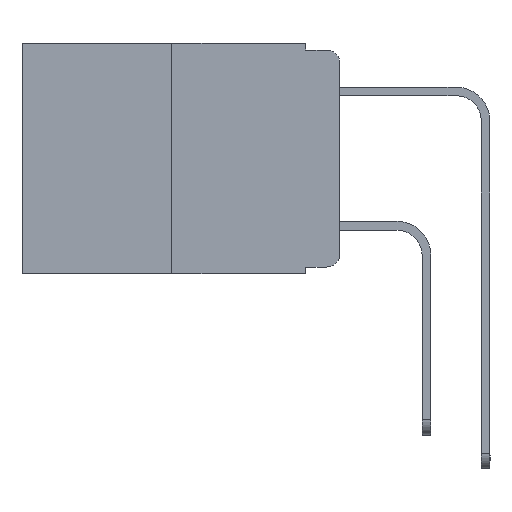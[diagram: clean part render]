
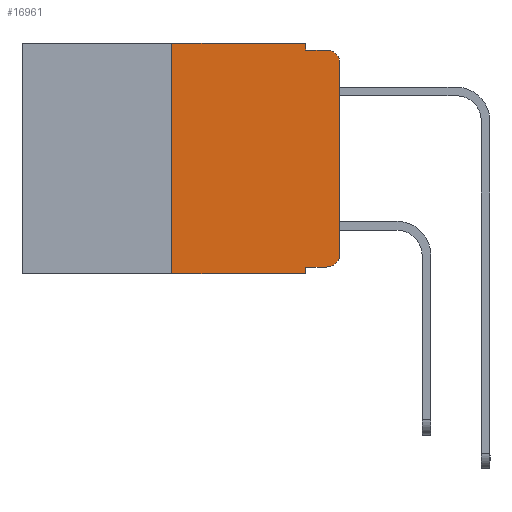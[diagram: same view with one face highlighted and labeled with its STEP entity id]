
A CAD part, left-side view. The second image highlights one B-rep face of the part: STEP entity #16961.
In plain terms, the highlighted planar face has unit normal (-1, 0, 0).
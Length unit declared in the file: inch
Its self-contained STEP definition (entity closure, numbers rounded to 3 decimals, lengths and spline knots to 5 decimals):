
#187 = VECTOR ( 'NONE', #9243, 39.37008 ) ;
#615 = VECTOR ( 'NONE', #16335, 39.37008 ) ;
#871 = DIRECTION ( 'NONE',  ( 0., 0., -1. ) ) ;
#934 = VERTEX_POINT ( 'NONE', #4813 ) ;
#1190 = CARTESIAN_POINT ( 'NONE',  ( 0., 0.051, -0.01 ) ) ;
#1217 = DIRECTION ( 'NONE',  ( 0., 0., -1. ) ) ;
#1298 = VERTEX_POINT ( 'NONE', #15268 ) ;
#1376 = CARTESIAN_POINT ( 'NONE',  ( 0., 0.25, 0. ) ) ;
#1393 = EDGE_CURVE ( 'NONE', #1298, #19591, #6084, .T. ) ;
#1877 = VERTEX_POINT ( 'NONE', #20705 ) ;
#2088 = LINE ( 'NONE', #20078, #187 ) ;
#2416 = DIRECTION ( 'NONE',  ( -1., 0., 0. ) ) ;
#2520 = VECTOR ( 'NONE', #14126, 39.37008 ) ;
#2699 = DIRECTION ( 'NONE',  ( 0., -1., 0. ) ) ;
#2867 = VECTOR ( 'NONE', #12453, 39.37008 ) ;
#3029 = AXIS2_PLACEMENT_3D ( 'NONE', #5043, #12288, #1217 ) ;
#4813 = CARTESIAN_POINT ( 'NONE',  ( 0., 0.02, -0.333 ) ) ;
#4962 = CARTESIAN_POINT ( 'NONE',  ( 0., 0.051, 0. ) ) ;
#5043 = CARTESIAN_POINT ( 'NONE',  ( 0., 0.02, -0.03 ) ) ;
#5522 = CARTESIAN_POINT ( 'NONE',  ( 0., 0.051, -0.333 ) ) ;
#5581 = DIRECTION ( 'NONE',  ( 0., 0., 1. ) ) ;
#5627 = EDGE_LOOP ( 'NONE', ( #15135, #21212, #17317, #17106, #16101, #19995, #16126, #22831, #17142, #9707 ) ) ;
#5900 = CIRCLE ( 'NONE', #16168, 0.02 ) ;
#5955 = CARTESIAN_POINT ( 'NONE',  ( 0., 0.051, -0.343 ) ) ;
#6084 = LINE ( 'NONE', #1190, #10367 ) ;
#7629 = VERTEX_POINT ( 'NONE', #4962 ) ;
#8186 = CARTESIAN_POINT ( 'NONE',  ( 0., 0.051, 0. ) ) ;
#8844 = EDGE_CURVE ( 'NONE', #12749, #22861, #19144, .T. ) ;
#8911 = EDGE_CURVE ( 'NONE', #12749, #1877, #23276, .T. ) ;
#8968 = EDGE_CURVE ( 'NONE', #1877, #7629, #23394, .T. ) ;
#9243 = DIRECTION ( 'NONE',  ( 0., 0., -1. ) ) ;
#9707 = ORIENTED_EDGE ( 'NONE', *, *, #16704, .T. ) ;
#9845 = LINE ( 'NONE', #8186, #22185 ) ;
#10367 = VECTOR ( 'NONE', #20855, 39.37008 ) ;
#10741 = LINE ( 'NONE', #16454, #615 ) ;
#10837 = AXIS2_PLACEMENT_3D ( 'NONE', #19213, #19673, #21328 ) ;
#11172 = CARTESIAN_POINT ( 'NONE',  ( 0., 0., 0. ) ) ;
#11943 = PLANE ( 'NONE',  #10837 ) ;
#12288 = DIRECTION ( 'NONE',  ( -1., 0., 0. ) ) ;
#12453 = DIRECTION ( 'NONE',  ( 0., -1., 0. ) ) ;
#12749 = VERTEX_POINT ( 'NONE', #22718 ) ;
#13586 = VECTOR ( 'NONE', #2699, 39.37008 ) ;
#14126 = DIRECTION ( 'NONE',  ( 0., 0., 1. ) ) ;
#14172 = VERTEX_POINT ( 'NONE', #14390 ) ;
#14390 = CARTESIAN_POINT ( 'NONE',  ( 0., 0., -0.03 ) ) ;
#15135 = ORIENTED_EDGE ( 'NONE', *, *, #15700, .T. ) ;
#15268 = CARTESIAN_POINT ( 'NONE',  ( 0., 0.051, -0.01 ) ) ;
#15700 = EDGE_CURVE ( 'NONE', #18930, #14172, #18546, .T. ) ;
#15900 = EDGE_CURVE ( 'NONE', #19671, #22861, #9845, .T. ) ;
#15982 = FACE_OUTER_BOUND ( 'NONE', #5627, .T. ) ;
#16101 = ORIENTED_EDGE ( 'NONE', *, *, #8968, .F. ) ;
#16126 = ORIENTED_EDGE ( 'NONE', *, *, #8844, .T. ) ;
#16144 = EDGE_CURVE ( 'NONE', #7629, #1298, #2088, .T. ) ;
#16168 = AXIS2_PLACEMENT_3D ( 'NONE', #22641, #2416, #871 ) ;
#16335 = DIRECTION ( 'NONE',  ( 0., -1., 0. ) ) ;
#16454 = CARTESIAN_POINT ( 'NONE',  ( 0., 0.051, -0.333 ) ) ;
#16704 = EDGE_CURVE ( 'NONE', #934, #18930, #5900, .T. ) ;
#16961 = ADVANCED_FACE ( 'NONE', ( #15982 ), #11943, .F. ) ;
#17106 = ORIENTED_EDGE ( 'NONE', *, *, #16144, .F. ) ;
#17142 = ORIENTED_EDGE ( 'NONE', *, *, #18292, .T. ) ;
#17317 = ORIENTED_EDGE ( 'NONE', *, *, #1393, .F. ) ;
#17812 = CARTESIAN_POINT ( 'NONE',  ( 0., 0.473, 0. ) ) ;
#18232 = CIRCLE ( 'NONE', #3029, 0.02 ) ;
#18292 = EDGE_CURVE ( 'NONE', #19671, #934, #10741, .T. ) ;
#18546 = LINE ( 'NONE', #11172, #18801 ) ;
#18801 = VECTOR ( 'NONE', #5581, 39.37008 ) ;
#18930 = VERTEX_POINT ( 'NONE', #22112 ) ;
#19018 = CARTESIAN_POINT ( 'NONE',  ( 0., 0.473, -0.343 ) ) ;
#19144 = LINE ( 'NONE', #19018, #13586 ) ;
#19213 = CARTESIAN_POINT ( 'NONE',  ( 0., 0.473, 0. ) ) ;
#19591 = VERTEX_POINT ( 'NONE', #21585 ) ;
#19671 = VERTEX_POINT ( 'NONE', #5522 ) ;
#19673 = DIRECTION ( 'NONE',  ( 1., 0., 0. ) ) ;
#19995 = ORIENTED_EDGE ( 'NONE', *, *, #8911, .F. ) ;
#20078 = CARTESIAN_POINT ( 'NONE',  ( 0., 0.051, 0. ) ) ;
#20705 = CARTESIAN_POINT ( 'NONE',  ( 0., 0.25, 0. ) ) ;
#20855 = DIRECTION ( 'NONE',  ( 0., -1., 0. ) ) ;
#21049 = DIRECTION ( 'NONE',  ( 0., 0., -1. ) ) ;
#21212 = ORIENTED_EDGE ( 'NONE', *, *, #22545, .T. ) ;
#21328 = DIRECTION ( 'NONE',  ( 0., 0., -1. ) ) ;
#21585 = CARTESIAN_POINT ( 'NONE',  ( 0., 0.02, -0.01 ) ) ;
#22112 = CARTESIAN_POINT ( 'NONE',  ( 0., 0., -0.313 ) ) ;
#22185 = VECTOR ( 'NONE', #21049, 39.37008 ) ;
#22545 = EDGE_CURVE ( 'NONE', #14172, #19591, #18232, .T. ) ;
#22641 = CARTESIAN_POINT ( 'NONE',  ( 0., 0.02, -0.313 ) ) ;
#22718 = CARTESIAN_POINT ( 'NONE',  ( 0., 0.25, -0.343 ) ) ;
#22831 = ORIENTED_EDGE ( 'NONE', *, *, #15900, .F. ) ;
#22861 = VERTEX_POINT ( 'NONE', #5955 ) ;
#23276 = LINE ( 'NONE', #1376, #2520 ) ;
#23394 = LINE ( 'NONE', #17812, #2867 ) ;
